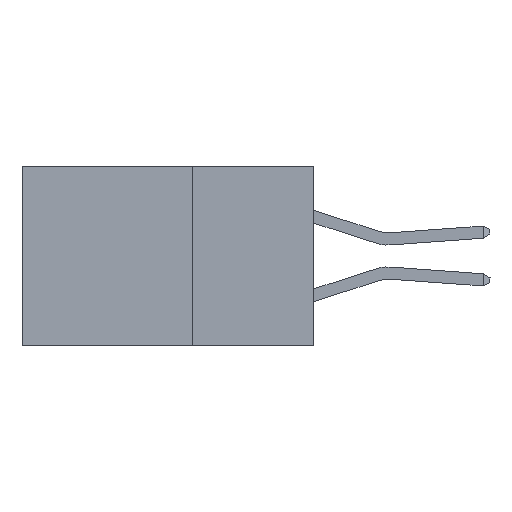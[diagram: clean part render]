
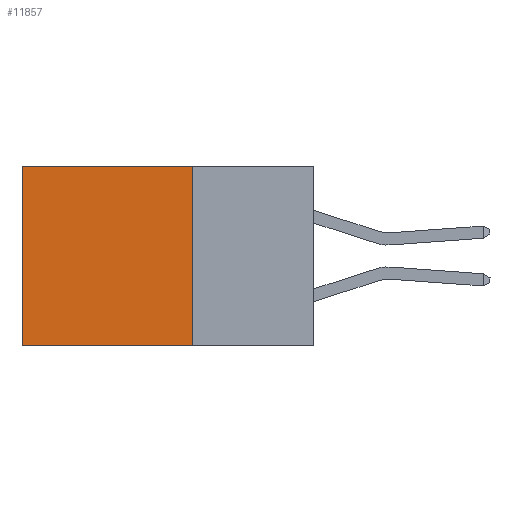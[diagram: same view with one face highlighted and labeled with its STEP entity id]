
A CAD part, left-side view. The second image highlights one B-rep face of the part: STEP entity #11857.
In plain terms, the highlighted planar face has unit normal (-1, 0, 0).
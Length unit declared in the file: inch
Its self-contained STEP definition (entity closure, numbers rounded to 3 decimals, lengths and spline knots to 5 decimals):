
#769 = CARTESIAN_POINT ( 'NONE',  ( 0.2875, 0.6, -0.37 ) ) ;
#978 = CARTESIAN_POINT ( 'NONE',  ( 0.2875, 0.25, 0. ) ) ;
#1214 = VECTOR ( 'NONE', #20749, 39.37008 ) ;
#1615 = ORIENTED_EDGE ( 'NONE', *, *, #16354, .F. ) ;
#3016 = CARTESIAN_POINT ( 'NONE',  ( 0.2875, 0.6, 0. ) ) ;
#3539 = LINE ( 'NONE', #17241, #14807 ) ;
#3708 = CARTESIAN_POINT ( 'NONE',  ( 0.2875, 0.25, 0. ) ) ;
#6220 = CARTESIAN_POINT ( 'NONE',  ( 0.2875, 0.25, 0. ) ) ;
#6320 = FACE_OUTER_BOUND ( 'NONE', #22152, .T. ) ;
#6465 = CARTESIAN_POINT ( 'NONE',  ( 0.2875, 0.25, -0.37 ) ) ;
#7045 = EDGE_CURVE ( 'NONE', #7423, #16401, #23217, .T. ) ;
#7423 = VERTEX_POINT ( 'NONE', #6220 ) ;
#8482 = DIRECTION ( 'NONE',  ( 0., 1., 0. ) ) ;
#8719 = PLANE ( 'NONE',  #12573 ) ;
#9141 = DIRECTION ( 'NONE',  ( 0., 1., 0. ) ) ;
#10343 = ORIENTED_EDGE ( 'NONE', *, *, #20928, .T. ) ;
#10488 = DIRECTION ( 'NONE',  ( 1., 0., 0. ) ) ;
#10633 = EDGE_CURVE ( 'NONE', #18278, #22917, #18458, .T. ) ;
#10868 = VECTOR ( 'NONE', #22731, 39.37008 ) ;
#11857 = ADVANCED_FACE ( 'NONE', ( #6320 ), #8719, .F. ) ;
#12573 = AXIS2_PLACEMENT_3D ( 'NONE', #978, #10488, #22123 ) ;
#12672 = ORIENTED_EDGE ( 'NONE', *, *, #7045, .F. ) ;
#12767 = CARTESIAN_POINT ( 'NONE',  ( 0.2875, 0.6, 0. ) ) ;
#13161 = ORIENTED_EDGE ( 'NONE', *, *, #10633, .T. ) ;
#14807 = VECTOR ( 'NONE', #9141, 39.37008 ) ;
#16354 = EDGE_CURVE ( 'NONE', #16401, #22917, #17986, .T. ) ;
#16401 = VERTEX_POINT ( 'NONE', #21535 ) ;
#17241 = CARTESIAN_POINT ( 'NONE',  ( 0.2875, 0.25, 0. ) ) ;
#17926 = VECTOR ( 'NONE', #8482, 39.37008 ) ;
#17986 = LINE ( 'NONE', #6465, #17926 ) ;
#18278 = VERTEX_POINT ( 'NONE', #3016 ) ;
#18458 = LINE ( 'NONE', #12767, #1214 ) ;
#20749 = DIRECTION ( 'NONE',  ( 0., 0., -1. ) ) ;
#20928 = EDGE_CURVE ( 'NONE', #7423, #18278, #3539, .T. ) ;
#21535 = CARTESIAN_POINT ( 'NONE',  ( 0.2875, 0.25, -0.37 ) ) ;
#22123 = DIRECTION ( 'NONE',  ( 0., 0., -1. ) ) ;
#22152 = EDGE_LOOP ( 'NONE', ( #13161, #1615, #12672, #10343 ) ) ;
#22731 = DIRECTION ( 'NONE',  ( 0., 0., -1. ) ) ;
#22917 = VERTEX_POINT ( 'NONE', #769 ) ;
#23217 = LINE ( 'NONE', #3708, #10868 ) ;
